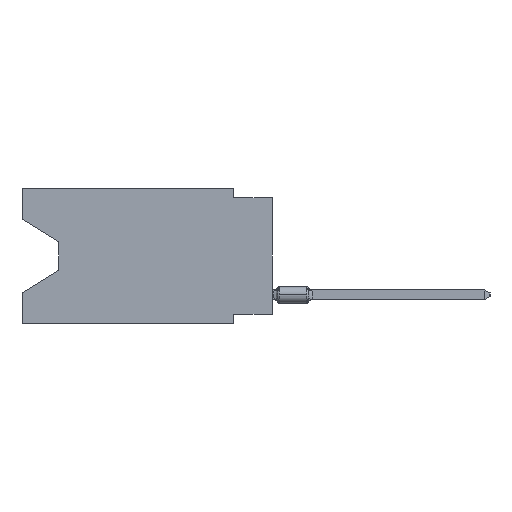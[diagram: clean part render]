
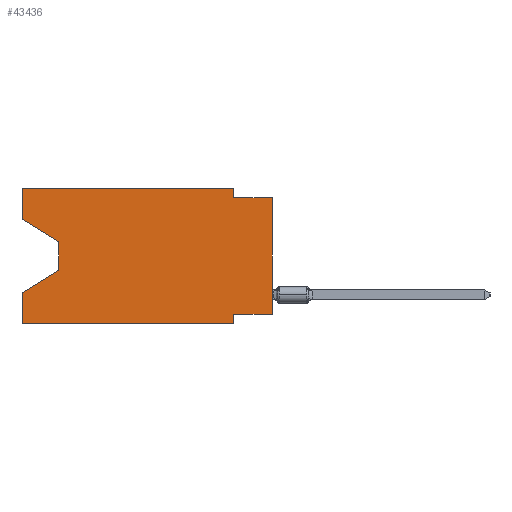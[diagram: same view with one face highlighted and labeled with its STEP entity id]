
A CAD part, left-side view. The second image highlights one B-rep face of the part: STEP entity #43436.
In plain terms, the highlighted planar face has unit normal (-1, 0, 0).
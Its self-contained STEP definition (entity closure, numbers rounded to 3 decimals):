
#677 = EDGE_CURVE ( 'NONE', #24725, #11502, #2026, .T. ) ;
#700 = ORIENTED_EDGE ( 'NONE', *, *, #33974, .T. ) ;
#758 = DIRECTION ( 'NONE',  ( 0., 0., -1. ) ) ;
#2026 = LINE ( 'NONE', #25619, #2808 ) ;
#2074 = ORIENTED_EDGE ( 'NONE', *, *, #14578, .F. ) ;
#2365 = VECTOR ( 'NONE', #8634, 1000. ) ;
#2607 = VERTEX_POINT ( 'NONE', #6213 ) ;
#2808 = VECTOR ( 'NONE', #26059, 1000. ) ;
#3295 = ORIENTED_EDGE ( 'NONE', *, *, #32600, .F. ) ;
#3824 = CARTESIAN_POINT ( 'NONE',  ( 0., 16.383, 0. ) ) ;
#4044 = EDGE_CURVE ( 'NONE', #41799, #13604, #25735, .T. ) ;
#4102 = CARTESIAN_POINT ( 'NONE',  ( 0., 2.54, -8.89 ) ) ;
#4106 = LINE ( 'NONE', #34661, #9862 ) ;
#4357 = VECTOR ( 'NONE', #40757, 1000. ) ;
#4827 = CARTESIAN_POINT ( 'NONE',  ( 0., 13.97, -5.385 ) ) ;
#5460 = EDGE_CURVE ( 'NONE', #27585, #23677, #44424, .T. ) ;
#6213 = CARTESIAN_POINT ( 'NONE',  ( 0., 0., -0.635 ) ) ;
#7593 = CARTESIAN_POINT ( 'NONE',  ( 0., 2.54, -0.635 ) ) ;
#7842 = EDGE_CURVE ( 'NONE', #13722, #2607, #14157, .T. ) ;
#8273 = VECTOR ( 'NONE', #34410, 1000. ) ;
#8634 = DIRECTION ( 'NONE',  ( 0., 0.855, -0.519 ) ) ;
#8981 = AXIS2_PLACEMENT_3D ( 'NONE', #24204, #13414, #33646 ) ;
#9862 = VECTOR ( 'NONE', #758, 1000. ) ;
#10484 = FACE_OUTER_BOUND ( 'NONE', #17918, .T. ) ;
#10539 = VERTEX_POINT ( 'NONE', #40673 ) ;
#11441 = VERTEX_POINT ( 'NONE', #11463 ) ;
#11463 = CARTESIAN_POINT ( 'NONE',  ( 0., 16.383, -8.89 ) ) ;
#11502 = VERTEX_POINT ( 'NONE', #31240 ) ;
#12180 = ORIENTED_EDGE ( 'NONE', *, *, #30060, .T. ) ;
#13414 = DIRECTION ( 'NONE',  ( 1., 0., 0. ) ) ;
#13604 = VERTEX_POINT ( 'NONE', #33684 ) ;
#13681 = CARTESIAN_POINT ( 'NONE',  ( 0., 16.383, 0. ) ) ;
#13722 = VERTEX_POINT ( 'NONE', #7593 ) ;
#14157 = LINE ( 'NONE', #37973, #14749 ) ;
#14341 = DIRECTION ( 'NONE',  ( 0., 0., 1. ) ) ;
#14558 = LINE ( 'NONE', #25565, #37913 ) ;
#14578 = EDGE_CURVE ( 'NONE', #11502, #21803, #16161, .T. ) ;
#14749 = VECTOR ( 'NONE', #35053, 1000. ) ;
#14885 = CARTESIAN_POINT ( 'NONE',  ( 0., 13.97, -5.385 ) ) ;
#15701 = ORIENTED_EDGE ( 'NONE', *, *, #27156, .F. ) ;
#16161 = LINE ( 'NONE', #40189, #33191 ) ;
#17049 = LINE ( 'NONE', #13681, #23379 ) ;
#17579 = LINE ( 'NONE', #38465, #32771 ) ;
#17918 = EDGE_LOOP ( 'NONE', ( #43982, #12180, #21804, #3295, #28626, #2074, #33694, #700, #33542, #31508, #31963, #15701 ) ) ;
#19092 = DIRECTION ( 'NONE',  ( 0., 0., -1. ) ) ;
#19566 = LINE ( 'NONE', #32622, #25815 ) ;
#20473 = CARTESIAN_POINT ( 'NONE',  ( 0., 16.383, -2.038 ) ) ;
#21803 = VERTEX_POINT ( 'NONE', #4102 ) ;
#21804 = ORIENTED_EDGE ( 'NONE', *, *, #4044, .T. ) ;
#23371 = CARTESIAN_POINT ( 'NONE',  ( 0., 13.97, -3.505 ) ) ;
#23379 = VECTOR ( 'NONE', #14341, 1000. ) ;
#23677 = VERTEX_POINT ( 'NONE', #39317 ) ;
#24204 = CARTESIAN_POINT ( 'NONE',  ( 0., 16.383, 0. ) ) ;
#24547 = DIRECTION ( 'NONE',  ( 0., 0., 1. ) ) ;
#24725 = VERTEX_POINT ( 'NONE', #35134 ) ;
#25565 = CARTESIAN_POINT ( 'NONE',  ( 0., 0., 0. ) ) ;
#25619 = CARTESIAN_POINT ( 'NONE',  ( 0., 0., -8.255 ) ) ;
#25735 = LINE ( 'NONE', #4827, #2365 ) ;
#25815 = VECTOR ( 'NONE', #29245, 1000. ) ;
#26059 = DIRECTION ( 'NONE',  ( 0., 1., 0. ) ) ;
#27156 = EDGE_CURVE ( 'NONE', #10539, #27585, #17579, .T. ) ;
#27585 = VERTEX_POINT ( 'NONE', #3824 ) ;
#28626 = ORIENTED_EDGE ( 'NONE', *, *, #41936, .T. ) ;
#29245 = DIRECTION ( 'NONE',  ( 0., -1., 0. ) ) ;
#30060 = EDGE_CURVE ( 'NONE', #37945, #41799, #4106, .T. ) ;
#30716 = DIRECTION ( 'NONE',  ( 0., -1., 0. ) ) ;
#31240 = CARTESIAN_POINT ( 'NONE',  ( 0., 2.54, -8.255 ) ) ;
#31508 = ORIENTED_EDGE ( 'NONE', *, *, #42624, .F. ) ;
#31963 = ORIENTED_EDGE ( 'NONE', *, *, #5460, .F. ) ;
#32076 = EDGE_CURVE ( 'NONE', #10539, #37945, #41574, .T. ) ;
#32600 = EDGE_CURVE ( 'NONE', #11441, #13604, #17049, .T. ) ;
#32622 = CARTESIAN_POINT ( 'NONE',  ( 0., 16.383, -8.89 ) ) ;
#32771 = VECTOR ( 'NONE', #24547, 1000. ) ;
#33191 = VECTOR ( 'NONE', #19092, 1000. ) ;
#33542 = ORIENTED_EDGE ( 'NONE', *, *, #7842, .F. ) ;
#33646 = DIRECTION ( 'NONE',  ( 0., 0., -1. ) ) ;
#33684 = CARTESIAN_POINT ( 'NONE',  ( 0., 16.383, -6.852 ) ) ;
#33694 = ORIENTED_EDGE ( 'NONE', *, *, #677, .F. ) ;
#33974 = EDGE_CURVE ( 'NONE', #24725, #2607, #14558, .T. ) ;
#34410 = DIRECTION ( 'NONE',  ( 0., -0.855, -0.519 ) ) ;
#34661 = CARTESIAN_POINT ( 'NONE',  ( 0., 13.97, -3.505 ) ) ;
#35053 = DIRECTION ( 'NONE',  ( 0., -1., 0. ) ) ;
#35134 = CARTESIAN_POINT ( 'NONE',  ( 0., 0., -8.255 ) ) ;
#37609 = LINE ( 'NONE', #44134, #4357 ) ;
#37913 = VECTOR ( 'NONE', #39254, 1000. ) ;
#37945 = VERTEX_POINT ( 'NONE', #23371 ) ;
#37973 = CARTESIAN_POINT ( 'NONE',  ( 0., 0., -0.635 ) ) ;
#38465 = CARTESIAN_POINT ( 'NONE',  ( 0., 16.383, 0. ) ) ;
#39044 = VECTOR ( 'NONE', #30716, 1000. ) ;
#39254 = DIRECTION ( 'NONE',  ( 0., 0., 1. ) ) ;
#39317 = CARTESIAN_POINT ( 'NONE',  ( 0., 2.54, 0. ) ) ;
#40189 = CARTESIAN_POINT ( 'NONE',  ( 0., 2.54, -8.89 ) ) ;
#40673 = CARTESIAN_POINT ( 'NONE',  ( 0., 16.383, -2.038 ) ) ;
#40757 = DIRECTION ( 'NONE',  ( 0., 0., -1. ) ) ;
#41574 = LINE ( 'NONE', #20473, #8273 ) ;
#41799 = VERTEX_POINT ( 'NONE', #14885 ) ;
#41936 = EDGE_CURVE ( 'NONE', #11441, #21803, #19566, .T. ) ;
#42624 = EDGE_CURVE ( 'NONE', #23677, #13722, #37609, .T. ) ;
#43436 = ADVANCED_FACE ( 'NONE', ( #10484 ), #43745, .F. ) ;
#43745 = PLANE ( 'NONE',  #8981 ) ;
#43982 = ORIENTED_EDGE ( 'NONE', *, *, #32076, .T. ) ;
#44134 = CARTESIAN_POINT ( 'NONE',  ( 0., 2.54, 0. ) ) ;
#44183 = CARTESIAN_POINT ( 'NONE',  ( 0., 16.383, 0. ) ) ;
#44424 = LINE ( 'NONE', #44183, #39044 ) ;
